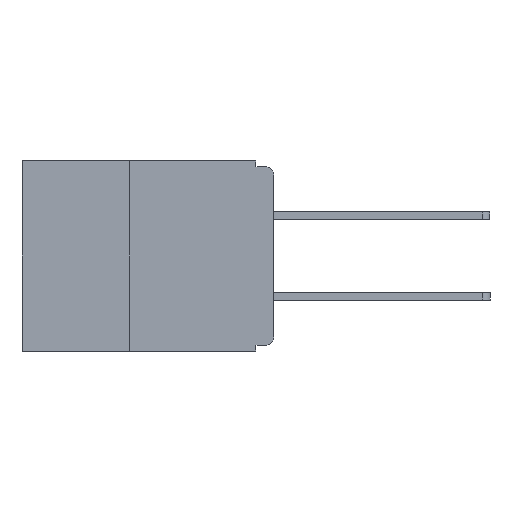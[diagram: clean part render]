
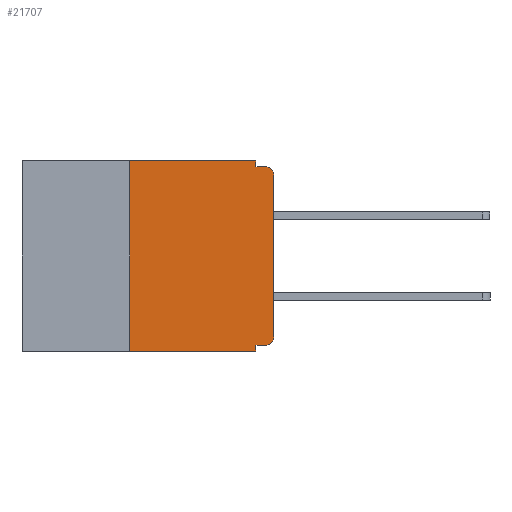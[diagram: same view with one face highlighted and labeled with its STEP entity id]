
A CAD part, left-side view. The second image highlights one B-rep face of the part: STEP entity #21707.
In plain terms, the highlighted planar face has unit normal (-1, 0, 0).
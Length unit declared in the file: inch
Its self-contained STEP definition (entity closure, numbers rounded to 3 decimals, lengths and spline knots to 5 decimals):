
#347 = VECTOR ( 'NONE', #11410, 39.37008 ) ;
#352 = CARTESIAN_POINT ( 'NONE',  ( 0., 0., 0. ) ) ;
#681 = VECTOR ( 'NONE', #9267, 39.37008 ) ;
#724 = ORIENTED_EDGE ( 'NONE', *, *, #14715, .T. ) ;
#754 = DIRECTION ( 'NONE',  ( 0., 1., 0. ) ) ;
#1082 = CARTESIAN_POINT ( 'NONE',  ( 0., 0.031, 0. ) ) ;
#1418 = ORIENTED_EDGE ( 'NONE', *, *, #16390, .F. ) ;
#1535 = EDGE_CURVE ( 'NONE', #6209, #4143, #20958, .T. ) ;
#2063 = DIRECTION ( 'NONE',  ( 0., 0., 1. ) ) ;
#2174 = ORIENTED_EDGE ( 'NONE', *, *, #11488, .F. ) ;
#2788 = ORIENTED_EDGE ( 'NONE', *, *, #5375, .T. ) ;
#3520 = ORIENTED_EDGE ( 'NONE', *, *, #9566, .T. ) ;
#3892 = LINE ( 'NONE', #9315, #20674 ) ;
#3900 = LINE ( 'NONE', #11668, #7960 ) ;
#4143 = VERTEX_POINT ( 'NONE', #19817 ) ;
#4960 = LINE ( 'NONE', #9579, #347 ) ;
#5127 = EDGE_LOOP ( 'NONE', ( #3520, #6790, #10440, #8564, #15751, #7915, #724, #1418, #2174, #2788 ) ) ;
#5375 = EDGE_CURVE ( 'NONE', #16351, #18904, #7852, .T. ) ;
#5508 = CARTESIAN_POINT ( 'NONE',  ( 0., 0., -0.025 ) ) ;
#5919 = VECTOR ( 'NONE', #6662, 39.37008 ) ;
#6209 = VERTEX_POINT ( 'NONE', #5508 ) ;
#6662 = DIRECTION ( 'NONE',  ( 0., 0., 1. ) ) ;
#6790 = ORIENTED_EDGE ( 'NONE', *, *, #1535, .T. ) ;
#6800 = CARTESIAN_POINT ( 'NONE',  ( 0., 0.437, 0. ) ) ;
#7814 = DIRECTION ( 'NONE',  ( -1., 0., 0. ) ) ;
#7852 = CIRCLE ( 'NONE', #14700, 0.015 ) ;
#7915 = ORIENTED_EDGE ( 'NONE', *, *, #13011, .F. ) ;
#7960 = VECTOR ( 'NONE', #18293, 39.37008 ) ;
#8306 = CARTESIAN_POINT ( 'NONE',  ( 0., 0., -0.305 ) ) ;
#8381 = DIRECTION ( 'NONE',  ( 0., 0., -1. ) ) ;
#8481 = DIRECTION ( 'NONE',  ( 0., 0., -1. ) ) ;
#8564 = ORIENTED_EDGE ( 'NONE', *, *, #18371, .F. ) ;
#9267 = DIRECTION ( 'NONE',  ( 0., -1., 0. ) ) ;
#9315 = CARTESIAN_POINT ( 'NONE',  ( 0., 0., -0.32 ) ) ;
#9566 = EDGE_CURVE ( 'NONE', #18904, #6209, #14716, .T. ) ;
#9579 = CARTESIAN_POINT ( 'NONE',  ( 0., 0.031, -0.33 ) ) ;
#9875 = VERTEX_POINT ( 'NONE', #1082 ) ;
#9910 = LINE ( 'NONE', #16825, #5919 ) ;
#9928 = FACE_OUTER_BOUND ( 'NONE', #5127, .T. ) ;
#10089 = LINE ( 'NONE', #16928, #18976 ) ;
#10148 = VECTOR ( 'NONE', #2063, 39.37008 ) ;
#10221 = DIRECTION ( 'NONE',  ( 0., 0., -1. ) ) ;
#10440 = ORIENTED_EDGE ( 'NONE', *, *, #18646, .F. ) ;
#11112 = VERTEX_POINT ( 'NONE', #16685 ) ;
#11205 = DIRECTION ( 'NONE',  ( 0., -1., 0. ) ) ;
#11410 = DIRECTION ( 'NONE',  ( 0., 0., -1. ) ) ;
#11488 = EDGE_CURVE ( 'NONE', #16351, #15400, #3892, .T. ) ;
#11668 = CARTESIAN_POINT ( 'NONE',  ( 0., 0.437, 0. ) ) ;
#11740 = DIRECTION ( 'NONE',  ( -1., 0., 0. ) ) ;
#11771 = DIRECTION ( 'NONE',  ( 0., 0., -1. ) ) ;
#11810 = VERTEX_POINT ( 'NONE', #16948 ) ;
#11938 = CARTESIAN_POINT ( 'NONE',  ( 0., 0.015, -0.305 ) ) ;
#12184 = CARTESIAN_POINT ( 'NONE',  ( 0., 0.25, 0. ) ) ;
#12521 = LINE ( 'NONE', #20995, #20213 ) ;
#13011 = EDGE_CURVE ( 'NONE', #11810, #19048, #9910, .T. ) ;
#13717 = VERTEX_POINT ( 'NONE', #18565 ) ;
#14700 = AXIS2_PLACEMENT_3D ( 'NONE', #11938, #11740, #11771 ) ;
#14715 = EDGE_CURVE ( 'NONE', #11810, #11112, #12521, .T. ) ;
#14716 = LINE ( 'NONE', #352, #10148 ) ;
#15210 = AXIS2_PLACEMENT_3D ( 'NONE', #16893, #7814, #8381 ) ;
#15400 = VERTEX_POINT ( 'NONE', #19534 ) ;
#15751 = ORIENTED_EDGE ( 'NONE', *, *, #18863, .F. ) ;
#16351 = VERTEX_POINT ( 'NONE', #18760 ) ;
#16390 = EDGE_CURVE ( 'NONE', #15400, #11112, #4960, .T. ) ;
#16685 = CARTESIAN_POINT ( 'NONE',  ( 0., 0.031, -0.33 ) ) ;
#16825 = CARTESIAN_POINT ( 'NONE',  ( 0., 0.25, -0.33 ) ) ;
#16893 = CARTESIAN_POINT ( 'NONE',  ( 0., 0.015, -0.025 ) ) ;
#16928 = CARTESIAN_POINT ( 'NONE',  ( 0., 0.031, 0. ) ) ;
#16948 = CARTESIAN_POINT ( 'NONE',  ( 0., 0.25, -0.33 ) ) ;
#16961 = PLANE ( 'NONE',  #17736 ) ;
#17684 = CARTESIAN_POINT ( 'NONE',  ( 0., 0., -0.01 ) ) ;
#17736 = AXIS2_PLACEMENT_3D ( 'NONE', #6800, #20140, #10221 ) ;
#18293 = DIRECTION ( 'NONE',  ( 0., -1., 0. ) ) ;
#18371 = EDGE_CURVE ( 'NONE', #9875, #13717, #10089, .T. ) ;
#18565 = CARTESIAN_POINT ( 'NONE',  ( 0., 0.031, -0.01 ) ) ;
#18646 = EDGE_CURVE ( 'NONE', #13717, #4143, #21417, .T. ) ;
#18760 = CARTESIAN_POINT ( 'NONE',  ( 0., 0.015, -0.32 ) ) ;
#18863 = EDGE_CURVE ( 'NONE', #19048, #9875, #3900, .T. ) ;
#18904 = VERTEX_POINT ( 'NONE', #8306 ) ;
#18976 = VECTOR ( 'NONE', #8481, 39.37008 ) ;
#19048 = VERTEX_POINT ( 'NONE', #12184 ) ;
#19534 = CARTESIAN_POINT ( 'NONE',  ( 0., 0.031, -0.32 ) ) ;
#19817 = CARTESIAN_POINT ( 'NONE',  ( 0., 0.015, -0.01 ) ) ;
#20140 = DIRECTION ( 'NONE',  ( 1., 0., 0. ) ) ;
#20213 = VECTOR ( 'NONE', #11205, 39.37008 ) ;
#20674 = VECTOR ( 'NONE', #754, 39.37008 ) ;
#20958 = CIRCLE ( 'NONE', #15210, 0.015 ) ;
#20995 = CARTESIAN_POINT ( 'NONE',  ( 0., 0.437, -0.33 ) ) ;
#21417 = LINE ( 'NONE', #17684, #681 ) ;
#21707 = ADVANCED_FACE ( 'NONE', ( #9928 ), #16961, .F. ) ;
